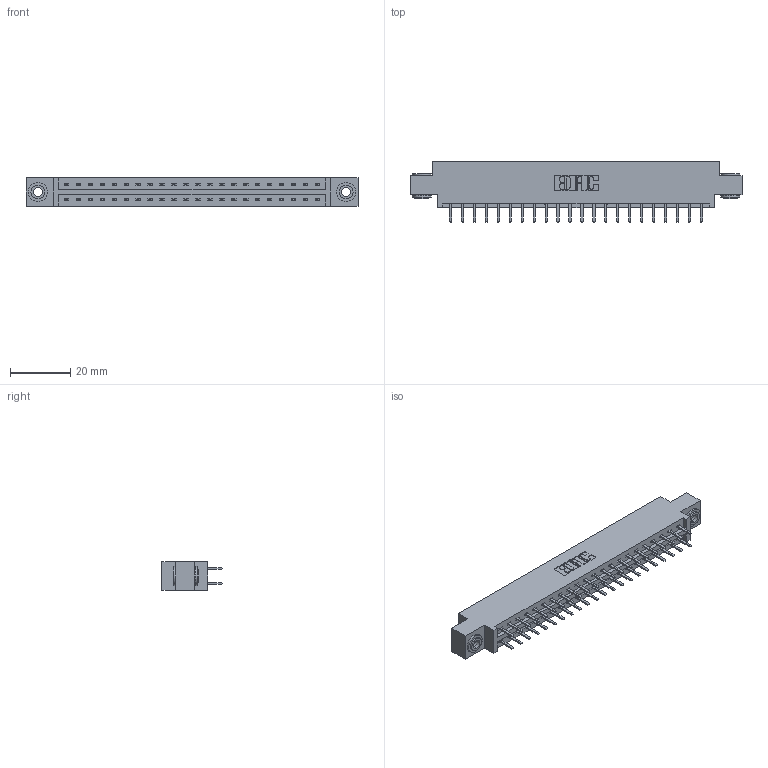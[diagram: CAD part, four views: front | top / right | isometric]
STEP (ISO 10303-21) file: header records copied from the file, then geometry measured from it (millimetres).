
FILE_DESCRIPTION (( 'STEP AP203' ), '1' );
FILE_NAME ('337-044-520-803.STEP', '2019-10-11T13:21:33', ( '' ), ( '' ), 'SwSTEP 2.0', 'SolidWorks 2016', '' );
FILE_SCHEMA (( 'CONFIG_CONTROL_DESIGN' ));
Length unit declared in the file: inch
Products named in the file (4): 345-292-001_345-293-120; 337-044-520-803; 337 Part_0.170 Offset - 0.156 Dia-TH; 345-250-002_345-250-002-102
Assembly tree (47 placements, depth 2):
  337-044-520-803
    337 Part_0.170 Offset - 0.156 Dia-TH
    345-292-001_345-293-120  x44
    345-250-002_345-250-002-102  x2
Bounding box: 110.19 x 20.02 x 9.4 mm (x, y, z)
Volume: 11228.5 mm3; surface area: 12776.7 mm2
Topology: 47 solids, 47 shells, 2708 faces, 7835 edges, 5102 vertices
Faces by surface type: plane 1844, cylinder 856, cone 8
Entity records: 20540 total; most frequent: CARTESIAN_POINT 3465, ORIENTED_EDGE 3382, DIRECTION 3005, EDGE_CURVE 1691, LINE 1535, VECTOR 1535, VERTEX_POINT 1122, AXIS2_PLACEMENT_3D 735
